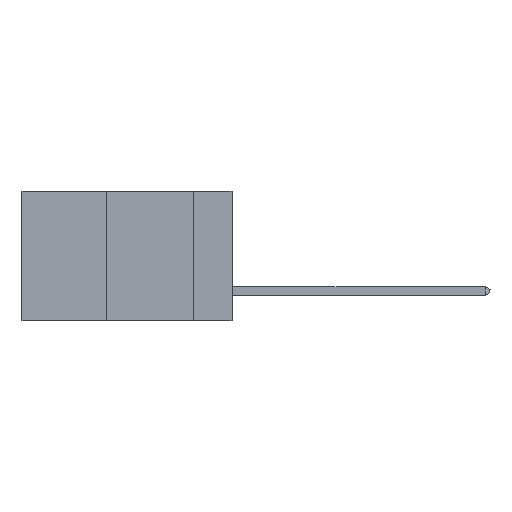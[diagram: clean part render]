
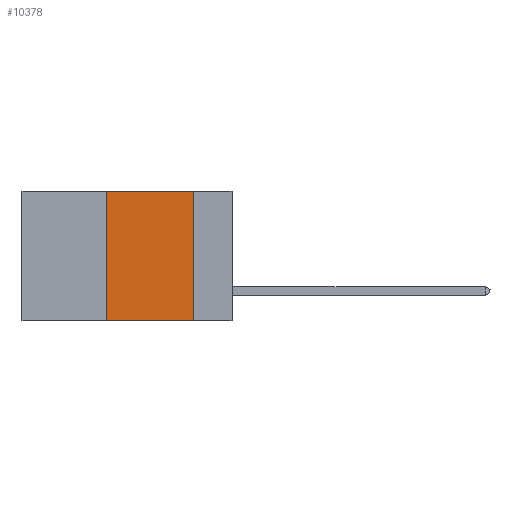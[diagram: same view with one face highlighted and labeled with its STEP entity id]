
A CAD part, left-side view. The second image highlights one B-rep face of the part: STEP entity #10378.
In plain terms, the highlighted planar face has unit normal (-1, 0, 0).
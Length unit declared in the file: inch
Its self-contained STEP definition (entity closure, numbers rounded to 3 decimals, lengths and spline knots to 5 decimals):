
#36 = CARTESIAN_POINT ( 'NONE',  ( 0., 0.6, 0. ) ) ;
#510 = FACE_OUTER_BOUND ( 'NONE', #4233, .T. ) ;
#520 = VECTOR ( 'NONE', #10279, 39.37008 ) ;
#602 = VERTEX_POINT ( 'NONE', #11120 ) ;
#1615 = CARTESIAN_POINT ( 'NONE',  ( 0., 0.36, -0.37 ) ) ;
#2234 = CARTESIAN_POINT ( 'NONE',  ( 0., 0.11, 0. ) ) ;
#2336 = ORIENTED_EDGE ( 'NONE', *, *, #2765, .F. ) ;
#2338 = EDGE_CURVE ( 'NONE', #2600, #8677, #7954, .T. ) ;
#2600 = VERTEX_POINT ( 'NONE', #5521 ) ;
#2765 = EDGE_CURVE ( 'NONE', #7093, #602, #2988, .T. ) ;
#2988 = LINE ( 'NONE', #4082, #520 ) ;
#3104 = LINE ( 'NONE', #36, #10507 ) ;
#3268 = VECTOR ( 'NONE', #10065, 39.37008 ) ;
#4082 = CARTESIAN_POINT ( 'NONE',  ( 0., 0.36, 0. ) ) ;
#4177 = CARTESIAN_POINT ( 'NONE',  ( 0., 0.6, -0.37 ) ) ;
#4233 = EDGE_LOOP ( 'NONE', ( #4313, #10457, #2336, #4339 ) ) ;
#4313 = ORIENTED_EDGE ( 'NONE', *, *, #2338, .F. ) ;
#4339 = ORIENTED_EDGE ( 'NONE', *, *, #9856, .T. ) ;
#4351 = EDGE_CURVE ( 'NONE', #602, #2600, #3104, .T. ) ;
#4480 = PLANE ( 'NONE',  #8940 ) ;
#5521 = CARTESIAN_POINT ( 'NONE',  ( 0., 0.11, 0. ) ) ;
#6820 = DIRECTION ( 'NONE',  ( 0., -1., 0. ) ) ;
#7093 = VERTEX_POINT ( 'NONE', #1615 ) ;
#7739 = DIRECTION ( 'NONE',  ( 1., 0., 0. ) ) ;
#7898 = CARTESIAN_POINT ( 'NONE',  ( 0., 0.6, 0. ) ) ;
#7954 = LINE ( 'NONE', #2234, #3268 ) ;
#8190 = DIRECTION ( 'NONE',  ( 0., -1., 0. ) ) ;
#8677 = VERTEX_POINT ( 'NONE', #10340 ) ;
#8908 = VECTOR ( 'NONE', #6820, 39.37008 ) ;
#8940 = AXIS2_PLACEMENT_3D ( 'NONE', #7898, #7739, #10455 ) ;
#9459 = LINE ( 'NONE', #4177, #8908 ) ;
#9856 = EDGE_CURVE ( 'NONE', #7093, #8677, #9459, .T. ) ;
#10065 = DIRECTION ( 'NONE',  ( 0., 0., -1. ) ) ;
#10279 = DIRECTION ( 'NONE',  ( 0., 0., 1. ) ) ;
#10340 = CARTESIAN_POINT ( 'NONE',  ( 0., 0.11, -0.37 ) ) ;
#10378 = ADVANCED_FACE ( 'NONE', ( #510 ), #4480, .F. ) ;
#10455 = DIRECTION ( 'NONE',  ( 0., 0., -1. ) ) ;
#10457 = ORIENTED_EDGE ( 'NONE', *, *, #4351, .F. ) ;
#10507 = VECTOR ( 'NONE', #8190, 39.37008 ) ;
#11120 = CARTESIAN_POINT ( 'NONE',  ( 0., 0.36, 0. ) ) ;
